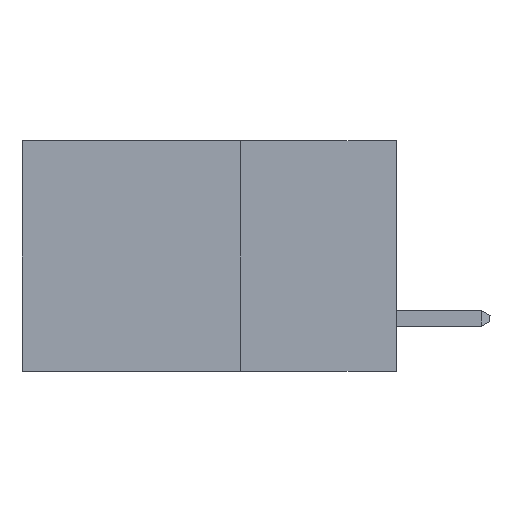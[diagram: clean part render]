
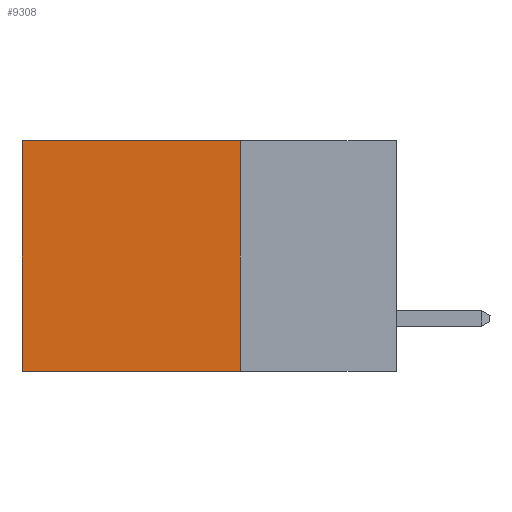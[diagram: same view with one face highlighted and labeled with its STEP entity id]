
A CAD part, left-side view. The second image highlights one B-rep face of the part: STEP entity #9308.
In plain terms, the highlighted planar face has unit normal (-1, 0, 0).
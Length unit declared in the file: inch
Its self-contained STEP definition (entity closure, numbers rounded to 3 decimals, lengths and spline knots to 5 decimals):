
#39 = CARTESIAN_POINT ( 'NONE',  ( 0.2615, 0.25, -0.37 ) ) ;
#238 = LINE ( 'NONE', #3167, #8921 ) ;
#331 = ORIENTED_EDGE ( 'NONE', *, *, #354, .F. ) ;
#354 = EDGE_CURVE ( 'NONE', #1556, #2742, #2902, .T. ) ;
#915 = PLANE ( 'NONE',  #5597 ) ;
#1466 = VECTOR ( 'NONE', #7417, 39.37008 ) ;
#1484 = DIRECTION ( 'NONE',  ( 0., 0., -1. ) ) ;
#1556 = VERTEX_POINT ( 'NONE', #5047 ) ;
#2037 = ORIENTED_EDGE ( 'NONE', *, *, #3826, .T. ) ;
#2045 = DIRECTION ( 'NONE',  ( 0., 0., -1. ) ) ;
#2253 = ORIENTED_EDGE ( 'NONE', *, *, #6116, .T. ) ;
#2363 = FACE_OUTER_BOUND ( 'NONE', #6744, .T. ) ;
#2474 = VECTOR ( 'NONE', #8663, 39.37008 ) ;
#2478 = LINE ( 'NONE', #5354, #1466 ) ;
#2523 = ORIENTED_EDGE ( 'NONE', *, *, #3244, .F. ) ;
#2742 = VERTEX_POINT ( 'NONE', #5058 ) ;
#2754 = CARTESIAN_POINT ( 'NONE',  ( 0.2615, 0.6, -0.37 ) ) ;
#2902 = LINE ( 'NONE', #7876, #2474 ) ;
#3167 = CARTESIAN_POINT ( 'NONE',  ( 0.2615, 0.25, -0.37 ) ) ;
#3244 = EDGE_CURVE ( 'NONE', #2742, #6032, #238, .T. ) ;
#3826 = EDGE_CURVE ( 'NONE', #6873, #6032, #9171, .T. ) ;
#5047 = CARTESIAN_POINT ( 'NONE',  ( 0.2615, 0.25, 0. ) ) ;
#5058 = CARTESIAN_POINT ( 'NONE',  ( 0.2615, 0.25, -0.37 ) ) ;
#5354 = CARTESIAN_POINT ( 'NONE',  ( 0.2615, 0.25, 0. ) ) ;
#5597 = AXIS2_PLACEMENT_3D ( 'NONE', #39, #7254, #1484 ) ;
#5860 = CARTESIAN_POINT ( 'NONE',  ( 0.2615, 0.6, 0. ) ) ;
#6032 = VERTEX_POINT ( 'NONE', #6803 ) ;
#6116 = EDGE_CURVE ( 'NONE', #1556, #6873, #2478, .T. ) ;
#6735 = VECTOR ( 'NONE', #2045, 39.37008 ) ;
#6744 = EDGE_LOOP ( 'NONE', ( #2037, #2523, #331, #2253 ) ) ;
#6803 = CARTESIAN_POINT ( 'NONE',  ( 0.2615, 0.6, -0.37 ) ) ;
#6873 = VERTEX_POINT ( 'NONE', #5860 ) ;
#7254 = DIRECTION ( 'NONE',  ( 1., 0., 0. ) ) ;
#7417 = DIRECTION ( 'NONE',  ( 0., 1., 0. ) ) ;
#7876 = CARTESIAN_POINT ( 'NONE',  ( 0.2615, 0.25, -0.37 ) ) ;
#8641 = DIRECTION ( 'NONE',  ( 0., 1., 0. ) ) ;
#8663 = DIRECTION ( 'NONE',  ( 0., 0., -1. ) ) ;
#8921 = VECTOR ( 'NONE', #8641, 39.37008 ) ;
#9171 = LINE ( 'NONE', #2754, #6735 ) ;
#9308 = ADVANCED_FACE ( 'NONE', ( #2363 ), #915, .F. ) ;
